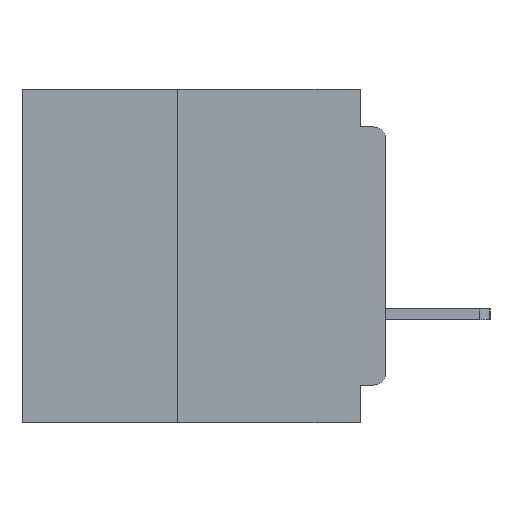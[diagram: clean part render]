
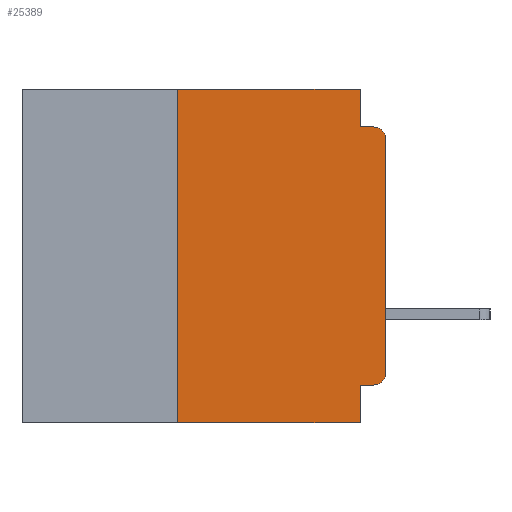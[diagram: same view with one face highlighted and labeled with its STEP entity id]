
A CAD part, left-side view. The second image highlights one B-rep face of the part: STEP entity #25389.
In plain terms, the highlighted planar face has unit normal (-1, 0, 0).
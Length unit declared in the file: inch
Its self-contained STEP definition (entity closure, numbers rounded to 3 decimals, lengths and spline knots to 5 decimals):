
#423 = VERTEX_POINT ( 'NONE', #8379 ) ;
#1085 = EDGE_CURVE ( 'NONE', #25622, #7976, #1263, .T. ) ;
#1109 = VECTOR ( 'NONE', #30484, 39.37008 ) ;
#1255 = ORIENTED_EDGE ( 'NONE', *, *, #17188, .F. ) ;
#1263 = LINE ( 'NONE', #37681, #11273 ) ;
#1551 = CARTESIAN_POINT ( 'NONE',  ( 0., 0.031, -0.4 ) ) ;
#1809 = ORIENTED_EDGE ( 'NONE', *, *, #39807, .T. ) ;
#1989 = CARTESIAN_POINT ( 'NONE',  ( 0., 0., -0.34 ) ) ;
#2411 = LINE ( 'NONE', #47353, #1109 ) ;
#3828 = EDGE_CURVE ( 'NONE', #423, #5340, #13677, .T. ) ;
#5340 = VERTEX_POINT ( 'NONE', #30331 ) ;
#6036 = CARTESIAN_POINT ( 'NONE',  ( 0., 0.031, 0. ) ) ;
#7976 = VERTEX_POINT ( 'NONE', #42284 ) ;
#8185 = CARTESIAN_POINT ( 'NONE',  ( 0., 0.437, -0.4 ) ) ;
#8379 = CARTESIAN_POINT ( 'NONE',  ( 0., 0.015, -0.355 ) ) ;
#9677 = PLANE ( 'NONE',  #31268 ) ;
#10329 = DIRECTION ( 'NONE',  ( 0., 0., -1. ) ) ;
#10346 = DIRECTION ( 'NONE',  ( 0., 0., -1. ) ) ;
#11273 = VECTOR ( 'NONE', #36795, 39.37008 ) ;
#11443 = ORIENTED_EDGE ( 'NONE', *, *, #50961, .T. ) ;
#12170 = EDGE_CURVE ( 'NONE', #40130, #29577, #40172, .T. ) ;
#12202 = VECTOR ( 'NONE', #25944, 39.37008 ) ;
#13480 = AXIS2_PLACEMENT_3D ( 'NONE', #39084, #13515, #43347 ) ;
#13515 = DIRECTION ( 'NONE',  ( -1., 0., 0. ) ) ;
#13677 = LINE ( 'NONE', #19637, #48960 ) ;
#14416 = ORIENTED_EDGE ( 'NONE', *, *, #24655, .F. ) ;
#16371 = CARTESIAN_POINT ( 'NONE',  ( 0., 0.25, -0.4 ) ) ;
#17116 = LINE ( 'NONE', #6036, #38444 ) ;
#17188 = EDGE_CURVE ( 'NONE', #41434, #41524, #34908, .T. ) ;
#17950 = EDGE_CURVE ( 'NONE', #5340, #47265, #50786, .T. ) ;
#18019 = ORIENTED_EDGE ( 'NONE', *, *, #12170, .T. ) ;
#18498 = AXIS2_PLACEMENT_3D ( 'NONE', #45134, #19657, #49375 ) ;
#19399 = DIRECTION ( 'NONE',  ( 0., 1., 0. ) ) ;
#19452 = VECTOR ( 'NONE', #55018, 39.37008 ) ;
#19637 = CARTESIAN_POINT ( 'NONE',  ( 0., 0., -0.355 ) ) ;
#19657 = DIRECTION ( 'NONE',  ( -1., 0., 0. ) ) ;
#20209 = CIRCLE ( 'NONE', #13480, 0.015 ) ;
#20623 = EDGE_CURVE ( 'NONE', #54462, #41434, #17116, .T. ) ;
#21256 = CARTESIAN_POINT ( 'NONE',  ( 0., 0., 0. ) ) ;
#22592 = DIRECTION ( 'NONE',  ( 0., 0., -1. ) ) ;
#24417 = ORIENTED_EDGE ( 'NONE', *, *, #20623, .F. ) ;
#24655 = EDGE_CURVE ( 'NONE', #7976, #54462, #2411, .T. ) ;
#25389 = ADVANCED_FACE ( 'NONE', ( #30408 ), #9677, .F. ) ;
#25587 = DIRECTION ( 'NONE',  ( 0., 0., 1. ) ) ;
#25622 = VERTEX_POINT ( 'NONE', #16371 ) ;
#25842 = ORIENTED_EDGE ( 'NONE', *, *, #17950, .F. ) ;
#25944 = DIRECTION ( 'NONE',  ( 0., -1., 0. ) ) ;
#26691 = CARTESIAN_POINT ( 'NONE',  ( 0., 0.437, 0. ) ) ;
#27714 = CIRCLE ( 'NONE', #18498, 0.015 ) ;
#29133 = CARTESIAN_POINT ( 'NONE',  ( 0., 0.031, -0.4 ) ) ;
#29404 = CARTESIAN_POINT ( 'NONE',  ( 0., 0.015, -0.045 ) ) ;
#29577 = VERTEX_POINT ( 'NONE', #41345 ) ;
#30331 = CARTESIAN_POINT ( 'NONE',  ( 0., 0.031, -0.355 ) ) ;
#30408 = FACE_OUTER_BOUND ( 'NONE', #35202, .T. ) ;
#30484 = DIRECTION ( 'NONE',  ( 0., -1., 0. ) ) ;
#30815 = LINE ( 'NONE', #8185, #19452 ) ;
#31168 = EDGE_CURVE ( 'NONE', #29577, #41524, #27714, .T. ) ;
#31268 = AXIS2_PLACEMENT_3D ( 'NONE', #26691, #48004, #22592 ) ;
#33100 = CARTESIAN_POINT ( 'NONE',  ( 0., 0.031, -0.045 ) ) ;
#34474 = CARTESIAN_POINT ( 'NONE',  ( 0., 0., -0.045 ) ) ;
#34908 = LINE ( 'NONE', #34474, #12202 ) ;
#35202 = EDGE_LOOP ( 'NONE', ( #18019, #52518, #1255, #24417, #14416, #53102, #1809, #25842, #39779, #11443 ) ) ;
#36795 = DIRECTION ( 'NONE',  ( 0., 0., 1. ) ) ;
#37681 = CARTESIAN_POINT ( 'NONE',  ( 0., 0.25, -0.4 ) ) ;
#38444 = VECTOR ( 'NONE', #10346, 39.37008 ) ;
#39084 = CARTESIAN_POINT ( 'NONE',  ( 0., 0.015, -0.34 ) ) ;
#39564 = VECTOR ( 'NONE', #10329, 39.37008 ) ;
#39779 = ORIENTED_EDGE ( 'NONE', *, *, #3828, .F. ) ;
#39807 = EDGE_CURVE ( 'NONE', #25622, #47265, #30815, .T. ) ;
#40130 = VERTEX_POINT ( 'NONE', #1989 ) ;
#40172 = LINE ( 'NONE', #21256, #50082 ) ;
#40336 = CARTESIAN_POINT ( 'NONE',  ( 0., 0.031, 0. ) ) ;
#41345 = CARTESIAN_POINT ( 'NONE',  ( 0., 0., -0.06 ) ) ;
#41434 = VERTEX_POINT ( 'NONE', #33100 ) ;
#41524 = VERTEX_POINT ( 'NONE', #29404 ) ;
#42284 = CARTESIAN_POINT ( 'NONE',  ( 0., 0.25, 0. ) ) ;
#43347 = DIRECTION ( 'NONE',  ( 0., 0., -1. ) ) ;
#45134 = CARTESIAN_POINT ( 'NONE',  ( 0., 0.015, -0.06 ) ) ;
#47265 = VERTEX_POINT ( 'NONE', #29133 ) ;
#47353 = CARTESIAN_POINT ( 'NONE',  ( 0., 0.437, 0. ) ) ;
#48004 = DIRECTION ( 'NONE',  ( 1., 0., 0. ) ) ;
#48960 = VECTOR ( 'NONE', #19399, 39.37008 ) ;
#49375 = DIRECTION ( 'NONE',  ( 0., 0., -1. ) ) ;
#50082 = VECTOR ( 'NONE', #25587, 39.37008 ) ;
#50786 = LINE ( 'NONE', #1551, #39564 ) ;
#50961 = EDGE_CURVE ( 'NONE', #423, #40130, #20209, .T. ) ;
#52518 = ORIENTED_EDGE ( 'NONE', *, *, #31168, .T. ) ;
#53102 = ORIENTED_EDGE ( 'NONE', *, *, #1085, .F. ) ;
#54462 = VERTEX_POINT ( 'NONE', #40336 ) ;
#55018 = DIRECTION ( 'NONE',  ( 0., -1., 0. ) ) ;
